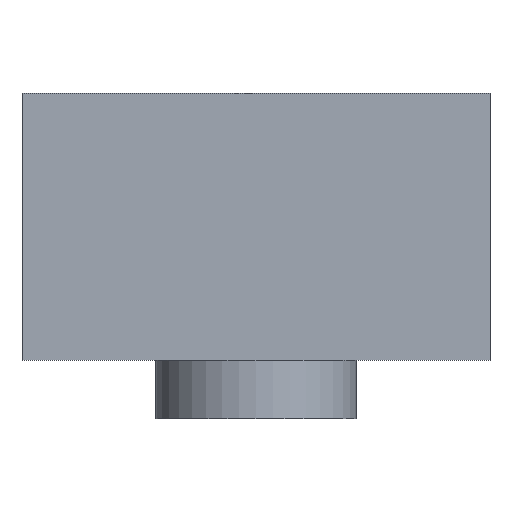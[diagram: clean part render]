
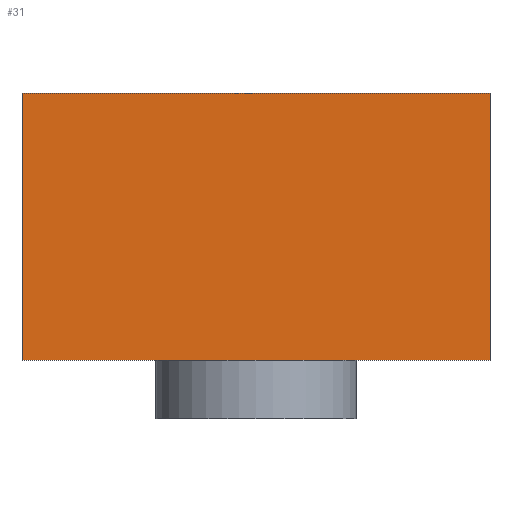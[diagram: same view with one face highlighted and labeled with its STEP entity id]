
A CAD part, front view. The second image highlights one B-rep face of the part: STEP entity #31.
In plain terms, the highlighted planar face has unit normal (0, -1, 0).
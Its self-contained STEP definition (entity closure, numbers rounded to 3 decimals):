
#31 = ADVANCED_FACE ( 'NONE', ( #748 ), #285, .F. ) ;
#33 = DIRECTION ( 'NONE',  ( 0., 0., -1. ) ) ;
#40 = VECTOR ( 'NONE', #50, 1000. ) ;
#50 = DIRECTION ( 'NONE',  ( -1., 0., 0. ) ) ;
#51 = CARTESIAN_POINT ( 'NONE',  ( 8.75, 45.305, -27.551 ) ) ;
#58 = ORIENTED_EDGE ( 'NONE', *, *, #645, .F. ) ;
#80 = EDGE_CURVE ( 'NONE', #223, #230, #741, .T. ) ;
#82 = ORIENTED_EDGE ( 'NONE', *, *, #80, .F. ) ;
#91 = CARTESIAN_POINT ( 'NONE',  ( 61.25, 45.305, -94.342 ) ) ;
#127 = AXIS2_PLACEMENT_3D ( 'NONE', #157, #557, #413 ) ;
#131 = CARTESIAN_POINT ( 'NONE',  ( 61.25, 45.305, -27.551 ) ) ;
#155 = CARTESIAN_POINT ( 'NONE',  ( 61.25, 45.305, -124.342 ) ) ;
#157 = CARTESIAN_POINT ( 'NONE',  ( 61.25, 45.305, -27.551 ) ) ;
#158 = CARTESIAN_POINT ( 'NONE',  ( 8.75, 45.305, -124.342 ) ) ;
#167 = DIRECTION ( 'NONE',  ( 0., 0., -1. ) ) ;
#211 = EDGE_LOOP ( 'NONE', ( #574, #58, #466, #82, #457 ) ) ;
#223 = VERTEX_POINT ( 'NONE', #527 ) ;
#230 = VERTEX_POINT ( 'NONE', #155 ) ;
#237 = EDGE_CURVE ( 'NONE', #230, #309, #441, .T. ) ;
#267 = LINE ( 'NONE', #51, #377 ) ;
#285 = PLANE ( 'NONE',  #127 ) ;
#309 = VERTEX_POINT ( 'NONE', #412 ) ;
#377 = VECTOR ( 'NONE', #33, 1000. ) ;
#409 = DIRECTION ( 'NONE',  ( -1., 0., 0. ) ) ;
#412 = CARTESIAN_POINT ( 'NONE',  ( 35., 45.305, -124.342 ) ) ;
#413 = DIRECTION ( 'NONE',  ( 0., 0., 1. ) ) ;
#429 = EDGE_CURVE ( 'NONE', #579, #740, #267, .T. ) ;
#441 = LINE ( 'NONE', #655, #488 ) ;
#457 = ORIENTED_EDGE ( 'NONE', *, *, #695, .T. ) ;
#458 = LINE ( 'NONE', #91, #548 ) ;
#460 = CARTESIAN_POINT ( 'NONE',  ( 61.25, 45.305, -124.342 ) ) ;
#466 = ORIENTED_EDGE ( 'NONE', *, *, #237, .F. ) ;
#488 = VECTOR ( 'NONE', #409, 1000. ) ;
#520 = CARTESIAN_POINT ( 'NONE',  ( 8.75, 45.305, -94.342 ) ) ;
#527 = CARTESIAN_POINT ( 'NONE',  ( 61.25, 45.305, -94.342 ) ) ;
#539 = LINE ( 'NONE', #460, #40 ) ;
#548 = VECTOR ( 'NONE', #641, 1000. ) ;
#557 = DIRECTION ( 'NONE',  ( 0., 1., 0. ) ) ;
#574 = ORIENTED_EDGE ( 'NONE', *, *, #429, .T. ) ;
#579 = VERTEX_POINT ( 'NONE', #520 ) ;
#641 = DIRECTION ( 'NONE',  ( -1., 0., 0. ) ) ;
#645 = EDGE_CURVE ( 'NONE', #309, #740, #539, .T. ) ;
#655 = CARTESIAN_POINT ( 'NONE',  ( 61.25, 45.305, -124.342 ) ) ;
#667 = VECTOR ( 'NONE', #167, 1000. ) ;
#695 = EDGE_CURVE ( 'NONE', #223, #579, #458, .T. ) ;
#740 = VERTEX_POINT ( 'NONE', #158 ) ;
#741 = LINE ( 'NONE', #131, #667 ) ;
#748 = FACE_OUTER_BOUND ( 'NONE', #211, .T. ) ;
